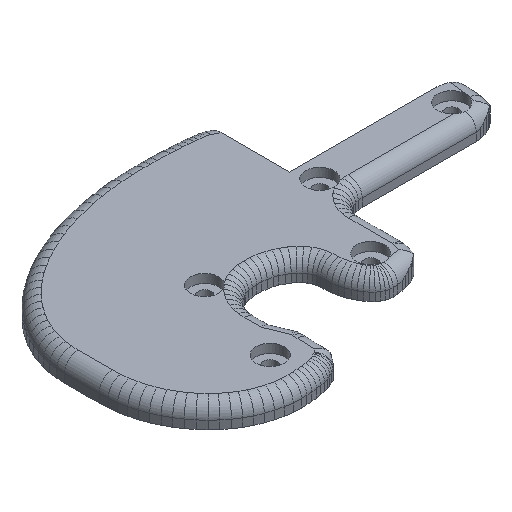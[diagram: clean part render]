
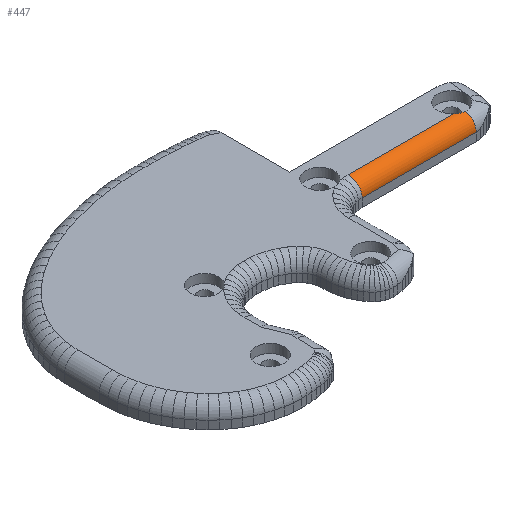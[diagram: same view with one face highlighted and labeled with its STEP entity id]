
A CAD part, isometric view. The second image highlights one B-rep face of the part: STEP entity #447.
In plain terms, the highlighted cylindrical face has radius 3.1 mm (diameter 6.2 mm), a partial arc.
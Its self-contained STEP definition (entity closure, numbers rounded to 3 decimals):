
#345=CARTESIAN_POINT('',(30.183,-3.142,4.902));
#346=VERTEX_POINT('',#345);
#359=CARTESIAN_POINT('',(30.28,-5.467,1.9));
#360=VERTEX_POINT('',#359);
#361=CARTESIAN_POINT('',(30.151,-2.367,1.9));
#362=DIRECTION('',(0.999,0.042,0.));
#363=DIRECTION('',(0.042,-0.999,0.));
#364=AXIS2_PLACEMENT_3D('',#361,#362,#363);
#365=ELLIPSE('',#364,3.103,3.1);
#366=EDGE_CURVE('',#346,#360,#365,.T.);
#405=CARTESIAN_POINT('',(-7.482,-2.367,1.9));
#406=DIRECTION('',(1.0,0.,0.0));
#407=DIRECTION('',(0.,-0.707,0.707));
#408=AXIS2_PLACEMENT_3D('',#405,#406,#407);
#409=CYLINDRICAL_SURFACE('',#408,3.1);
#410=CARTESIAN_POINT('',(4.187,-5.467,1.9));
#411=VERTEX_POINT('',#410);
#412=CARTESIAN_POINT('',(4.187,-5.467,1.9));
#413=DIRECTION('',(1.0,0.0,0.0));
#414=VECTOR('',#413,26.093);
#415=LINE('',#412,#414);
#416=EDGE_CURVE('',#411,#360,#415,.T.);
#417=ORIENTED_EDGE('',*,*,#416,.T.);
#418=ORIENTED_EDGE('',*,*,#366,.F.);
#419=CARTESIAN_POINT('',(28.172,-2.367,5.0));
#420=VERTEX_POINT('',#419);
#421=CARTESIAN_POINT('',(30.183,-3.142,4.902));
#422=CARTESIAN_POINT('',(29.69,-3.127,4.905));
#423=CARTESIAN_POINT('',(29.186,-2.995,4.945));
#424=CARTESIAN_POINT('',(28.538,-2.647,4.989));
#425=CARTESIAN_POINT('',(28.346,-2.515,5.0));
#426=CARTESIAN_POINT('',(28.172,-2.367,5.0));
#427=B_SPLINE_CURVE_WITH_KNOTS('',3,(#421,#422,#423,#424,#425,#426),.UNSPECIFIED.,.F.,.U.,(4,2,4),(0.01,0.157,0.224),.UNSPECIFIED.);
#428=EDGE_CURVE('',#346,#420,#427,.T.);
#429=ORIENTED_EDGE('',*,*,#428,.T.);
#430=CARTESIAN_POINT('',(4.052,-2.367,5.0));
#431=VERTEX_POINT('',#430);
#432=CARTESIAN_POINT('',(28.172,-2.367,5.0));
#433=DIRECTION('',(-1.0,0.0,0.0));
#434=VECTOR('',#433,24.12);
#435=LINE('',#432,#434);
#436=EDGE_CURVE('',#420,#431,#435,.T.);
#437=ORIENTED_EDGE('',*,*,#436,.T.);
#438=CARTESIAN_POINT('',(4.052,-2.367,1.9));
#439=DIRECTION('',(0.999,0.043,0.));
#440=DIRECTION('',(-0.043,0.999,0.));
#441=AXIS2_PLACEMENT_3D('',#438,#439,#440);
#442=ELLIPSE('',#441,3.103,3.1);
#443=EDGE_CURVE('',#431,#411,#442,.T.);
#444=ORIENTED_EDGE('',*,*,#443,.T.);
#445=EDGE_LOOP('',(#417,#418,#429,#437,#444));
#446=FACE_OUTER_BOUND('',#445,.T.);
#447=ADVANCED_FACE('',(#446),#409,.T.);
